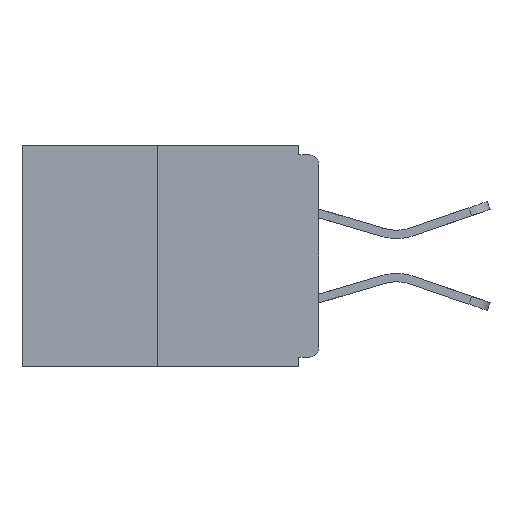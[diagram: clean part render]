
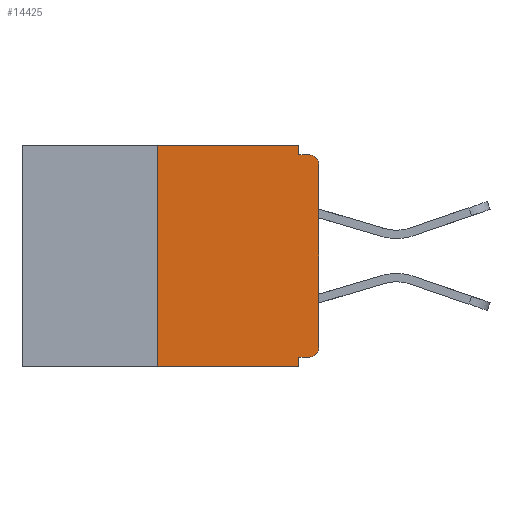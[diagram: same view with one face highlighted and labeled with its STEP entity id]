
A CAD part, left-side view. The second image highlights one B-rep face of the part: STEP entity #14425.
In plain terms, the highlighted planar face has unit normal (-1, 0, 0).
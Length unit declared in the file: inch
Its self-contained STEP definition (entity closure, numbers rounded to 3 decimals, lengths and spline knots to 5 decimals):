
#98 = CARTESIAN_POINT ( 'NONE',  ( 0., 0.015, -0.03 ) ) ;
#515 = ORIENTED_EDGE ( 'NONE', *, *, #3657, .F. ) ;
#811 = VERTEX_POINT ( 'NONE', #13652 ) ;
#933 = EDGE_CURVE ( 'NONE', #18526, #5899, #16932, .T. ) ;
#1316 = VECTOR ( 'NONE', #7344, 39.37008 ) ;
#1333 = CIRCLE ( 'NONE', #12437, 0.015 ) ;
#1349 = CIRCLE ( 'NONE', #4177, 0.015 ) ;
#1619 = EDGE_CURVE ( 'NONE', #5899, #1756, #10634, .T. ) ;
#1756 = VERTEX_POINT ( 'NONE', #13714 ) ;
#1848 = FACE_OUTER_BOUND ( 'NONE', #7711, .T. ) ;
#1989 = ORIENTED_EDGE ( 'NONE', *, *, #2289, .T. ) ;
#2230 = EDGE_CURVE ( 'NONE', #4895, #18830, #1333, .T. ) ;
#2289 = EDGE_CURVE ( 'NONE', #811, #1756, #1349, .T. ) ;
#2810 = CARTESIAN_POINT ( 'NONE',  ( 0., 0.46, -0.343 ) ) ;
#3238 = DIRECTION ( 'NONE',  ( 0., 0., -1. ) ) ;
#3657 = EDGE_CURVE ( 'NONE', #13887, #15297, #14851, .T. ) ;
#4177 = AXIS2_PLACEMENT_3D ( 'NONE', #98, #6418, #18150 ) ;
#4577 = CARTESIAN_POINT ( 'NONE',  ( 0., 0., 0. ) ) ;
#4644 = DIRECTION ( 'NONE',  ( -1., 0., 0. ) ) ;
#4723 = LINE ( 'NONE', #8002, #14028 ) ;
#4753 = VECTOR ( 'NONE', #16350, 39.37008 ) ;
#4776 = ORIENTED_EDGE ( 'NONE', *, *, #16101, .T. ) ;
#4795 = DIRECTION ( 'NONE',  ( 0., 0., -1. ) ) ;
#4895 = VERTEX_POINT ( 'NONE', #10121 ) ;
#5029 = CARTESIAN_POINT ( 'NONE',  ( 0., 0.25, -0.343 ) ) ;
#5078 = CARTESIAN_POINT ( 'NONE',  ( 0., 0.031, -0.343 ) ) ;
#5666 = EDGE_CURVE ( 'NONE', #4895, #6811, #6214, .T. ) ;
#5899 = VERTEX_POINT ( 'NONE', #14948 ) ;
#6214 = LINE ( 'NONE', #18327, #10035 ) ;
#6418 = DIRECTION ( 'NONE',  ( -1., 0., 0. ) ) ;
#6659 = EDGE_CURVE ( 'NONE', #13887, #9330, #14759, .T. ) ;
#6733 = AXIS2_PLACEMENT_3D ( 'NONE', #14164, #16838, #9321 ) ;
#6791 = VECTOR ( 'NONE', #4795, 39.37008 ) ;
#6811 = VERTEX_POINT ( 'NONE', #15531 ) ;
#7055 = CARTESIAN_POINT ( 'NONE',  ( 0., 0., -0.313 ) ) ;
#7344 = DIRECTION ( 'NONE',  ( 0., -1., 0. ) ) ;
#7711 = EDGE_LOOP ( 'NONE', ( #10440, #515, #8280, #10308, #8779, #18236, #4776, #1989, #18071, #16113 ) ) ;
#7906 = CARTESIAN_POINT ( 'NONE',  ( 0., 0.015, -0.313 ) ) ;
#8002 = CARTESIAN_POINT ( 'NONE',  ( 0., 0.46, 0. ) ) ;
#8280 = ORIENTED_EDGE ( 'NONE', *, *, #6659, .T. ) ;
#8779 = ORIENTED_EDGE ( 'NONE', *, *, #5666, .F. ) ;
#9321 = DIRECTION ( 'NONE',  ( 0., 0., -1. ) ) ;
#9330 = VERTEX_POINT ( 'NONE', #18093 ) ;
#9364 = VECTOR ( 'NONE', #12062, 39.37008 ) ;
#9372 = EDGE_CURVE ( 'NONE', #6811, #9330, #11049, .T. ) ;
#10035 = VECTOR ( 'NONE', #12962, 39.37008 ) ;
#10121 = CARTESIAN_POINT ( 'NONE',  ( 0., 0.015, -0.328 ) ) ;
#10308 = ORIENTED_EDGE ( 'NONE', *, *, #9372, .F. ) ;
#10332 = DIRECTION ( 'NONE',  ( 0., 0., 1. ) ) ;
#10440 = ORIENTED_EDGE ( 'NONE', *, *, #14382, .F. ) ;
#10634 = LINE ( 'NONE', #13412, #1316 ) ;
#10800 = VECTOR ( 'NONE', #10332, 39.37008 ) ;
#11049 = LINE ( 'NONE', #5078, #6791 ) ;
#11062 = CARTESIAN_POINT ( 'NONE',  ( 0., 0.031, 0. ) ) ;
#11076 = PLANE ( 'NONE',  #6733 ) ;
#12062 = DIRECTION ( 'NONE',  ( 0., -1., 0. ) ) ;
#12437 = AXIS2_PLACEMENT_3D ( 'NONE', #7906, #4644, #3238 ) ;
#12962 = DIRECTION ( 'NONE',  ( 0., 1., 0. ) ) ;
#13412 = CARTESIAN_POINT ( 'NONE',  ( 0., 0., -0.015 ) ) ;
#13483 = CARTESIAN_POINT ( 'NONE',  ( 0., 0.25, 0. ) ) ;
#13652 = CARTESIAN_POINT ( 'NONE',  ( 0., 0., -0.03 ) ) ;
#13714 = CARTESIAN_POINT ( 'NONE',  ( 0., 0.015, -0.015 ) ) ;
#13887 = VERTEX_POINT ( 'NONE', #5029 ) ;
#14028 = VECTOR ( 'NONE', #17237, 39.37008 ) ;
#14050 = DIRECTION ( 'NONE',  ( 0., 0., -1. ) ) ;
#14164 = CARTESIAN_POINT ( 'NONE',  ( 0., 0.46, 0. ) ) ;
#14382 = EDGE_CURVE ( 'NONE', #15297, #18526, #4723, .T. ) ;
#14425 = ADVANCED_FACE ( 'NONE', ( #1848 ), #11076, .F. ) ;
#14759 = LINE ( 'NONE', #2810, #9364 ) ;
#14851 = LINE ( 'NONE', #19542, #4753 ) ;
#14948 = CARTESIAN_POINT ( 'NONE',  ( 0., 0.031, -0.015 ) ) ;
#15019 = VECTOR ( 'NONE', #14050, 39.37008 ) ;
#15297 = VERTEX_POINT ( 'NONE', #13483 ) ;
#15317 = LINE ( 'NONE', #4577, #10800 ) ;
#15531 = CARTESIAN_POINT ( 'NONE',  ( 0., 0.031, -0.328 ) ) ;
#16101 = EDGE_CURVE ( 'NONE', #18830, #811, #15317, .T. ) ;
#16113 = ORIENTED_EDGE ( 'NONE', *, *, #933, .F. ) ;
#16350 = DIRECTION ( 'NONE',  ( 0., 0., 1. ) ) ;
#16838 = DIRECTION ( 'NONE',  ( 1., 0., 0. ) ) ;
#16932 = LINE ( 'NONE', #11062, #15019 ) ;
#17237 = DIRECTION ( 'NONE',  ( 0., -1., 0. ) ) ;
#18071 = ORIENTED_EDGE ( 'NONE', *, *, #1619, .F. ) ;
#18093 = CARTESIAN_POINT ( 'NONE',  ( 0., 0.031, -0.343 ) ) ;
#18150 = DIRECTION ( 'NONE',  ( 0., 0., -1. ) ) ;
#18236 = ORIENTED_EDGE ( 'NONE', *, *, #2230, .T. ) ;
#18327 = CARTESIAN_POINT ( 'NONE',  ( 0., 0., -0.328 ) ) ;
#18526 = VERTEX_POINT ( 'NONE', #19551 ) ;
#18830 = VERTEX_POINT ( 'NONE', #7055 ) ;
#19542 = CARTESIAN_POINT ( 'NONE',  ( 0., 0.25, 0. ) ) ;
#19551 = CARTESIAN_POINT ( 'NONE',  ( 0., 0.031, 0. ) ) ;
